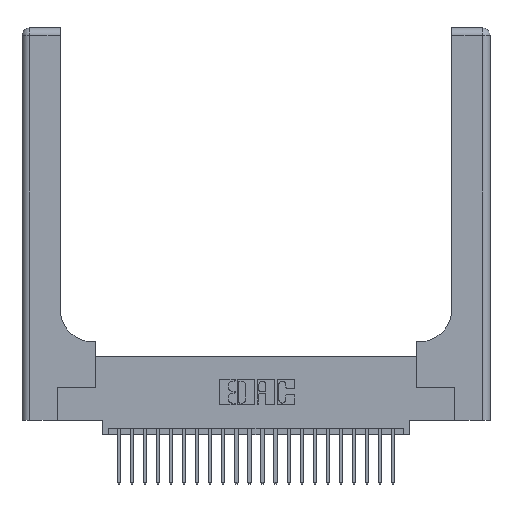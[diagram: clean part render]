
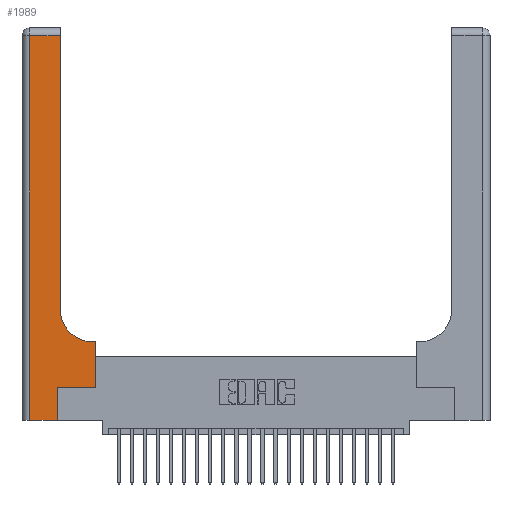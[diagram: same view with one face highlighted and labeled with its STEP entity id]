
A CAD part, top view. The second image highlights one B-rep face of the part: STEP entity #1989.
In plain terms, the highlighted planar face has unit normal (0, 0, 1).
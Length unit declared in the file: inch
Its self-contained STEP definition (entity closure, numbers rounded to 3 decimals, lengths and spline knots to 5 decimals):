
#318 = ORIENTED_EDGE ( 'NONE', *, *, #20393, .T. ) ;
#329 = CARTESIAN_POINT ( 'NONE',  ( 0.06, 0., 0.37 ) ) ;
#740 = EDGE_LOOP ( 'NONE', ( #21335, #24756, #16687, #18227, #22793, #7825, #9470, #23939, #318 ) ) ;
#787 = VECTOR ( 'NONE', #19542, 39.37008 ) ;
#1242 = VECTOR ( 'NONE', #10625, 39.37008 ) ;
#1989 = ADVANCED_FACE ( 'NONE', ( #13441 ), #8271, .F. ) ;
#2045 = LINE ( 'NONE', #21163, #17062 ) ;
#2426 = LINE ( 'NONE', #8465, #8575 ) ;
#2751 = VERTEX_POINT ( 'NONE', #9185 ) ;
#2783 = LINE ( 'NONE', #15528, #7411 ) ;
#2804 = EDGE_CURVE ( 'NONE', #16845, #6599, #2045, .T. ) ;
#3666 = CARTESIAN_POINT ( 'NONE',  ( 0.5585, 0.6, 0.37 ) ) ;
#4493 = EDGE_CURVE ( 'NONE', #8840, #17363, #17584, .T. ) ;
#4941 = EDGE_CURVE ( 'NONE', #7949, #16845, #2426, .T. ) ;
#5224 = VECTOR ( 'NONE', #7273, 39.37008 ) ;
#6599 = VERTEX_POINT ( 'NONE', #3666 ) ;
#6716 = DIRECTION ( 'NONE',  ( 0., 1., 0. ) ) ;
#7273 = DIRECTION ( 'NONE',  ( 0., -1., 0. ) ) ;
#7375 = EDGE_CURVE ( 'NONE', #10567, #2751, #8909, .T. ) ;
#7411 = VECTOR ( 'NONE', #21808, 39.37008 ) ;
#7825 = ORIENTED_EDGE ( 'NONE', *, *, #4941, .T. ) ;
#7949 = VERTEX_POINT ( 'NONE', #18211 ) ;
#8143 = LINE ( 'NONE', #21383, #787 ) ;
#8271 = PLANE ( 'NONE',  #23781 ) ;
#8465 = CARTESIAN_POINT ( 'NONE',  ( 0.269, 0.25, 0.37 ) ) ;
#8575 = VECTOR ( 'NONE', #18218, 39.37008 ) ;
#8693 = DIRECTION ( 'NONE',  ( 0., 0., -1. ) ) ;
#8840 = VERTEX_POINT ( 'NONE', #329 ) ;
#8909 = LINE ( 'NONE', #24203, #1242 ) ;
#9185 = CARTESIAN_POINT ( 'NONE',  ( 0.06, 2.94, 0.37 ) ) ;
#9470 = ORIENTED_EDGE ( 'NONE', *, *, #2804, .T. ) ;
#10244 = CARTESIAN_POINT ( 'NONE',  ( 0., 3., 0.37 ) ) ;
#10567 = VERTEX_POINT ( 'NONE', #21222 ) ;
#10625 = DIRECTION ( 'NONE',  ( -1., 0., 0. ) ) ;
#10696 = CARTESIAN_POINT ( 'NONE',  ( 0.269, 0., 0.37 ) ) ;
#12660 = CARTESIAN_POINT ( 'NONE',  ( 0., 0., 0.37 ) ) ;
#12858 = CARTESIAN_POINT ( 'NONE',  ( 0.5585, 0.25, 0.37 ) ) ;
#12900 = EDGE_CURVE ( 'NONE', #17363, #7949, #2783, .T. ) ;
#13174 = CARTESIAN_POINT ( 'NONE',  ( 0.06, 3., 0.37 ) ) ;
#13441 = FACE_OUTER_BOUND ( 'NONE', #740, .T. ) ;
#14233 = DIRECTION ( 'NONE',  ( 0., 0., -1. ) ) ;
#15145 = VECTOR ( 'NONE', #20596, 39.37008 ) ;
#15268 = LINE ( 'NONE', #18448, #17092 ) ;
#15528 = CARTESIAN_POINT ( 'NONE',  ( 0.269, 0., 0.37 ) ) ;
#16527 = EDGE_CURVE ( 'NONE', #6599, #24221, #8143, .T. ) ;
#16687 = ORIENTED_EDGE ( 'NONE', *, *, #18716, .T. ) ;
#16845 = VERTEX_POINT ( 'NONE', #12858 ) ;
#17062 = VECTOR ( 'NONE', #17097, 39.37008 ) ;
#17092 = VECTOR ( 'NONE', #6716, 39.37008 ) ;
#17097 = DIRECTION ( 'NONE',  ( 0., 1., 0. ) ) ;
#17363 = VERTEX_POINT ( 'NONE', #10696 ) ;
#17584 = LINE ( 'NONE', #12660, #15145 ) ;
#18211 = CARTESIAN_POINT ( 'NONE',  ( 0.269, 0.25, 0.37 ) ) ;
#18218 = DIRECTION ( 'NONE',  ( 1., 0., 0. ) ) ;
#18227 = ORIENTED_EDGE ( 'NONE', *, *, #4493, .T. ) ;
#18448 = CARTESIAN_POINT ( 'NONE',  ( 0.2915, 3., 0.37 ) ) ;
#18716 = EDGE_CURVE ( 'NONE', #2751, #8840, #25095, .T. ) ;
#18780 = AXIS2_PLACEMENT_3D ( 'NONE', #23960, #14233, #21905 ) ;
#19542 = DIRECTION ( 'NONE',  ( -1., 0., 0. ) ) ;
#20393 = EDGE_CURVE ( 'NONE', #24221, #23687, #23119, .T. ) ;
#20596 = DIRECTION ( 'NONE',  ( 1., 0., 0. ) ) ;
#21038 = CARTESIAN_POINT ( 'NONE',  ( 0.2915, 0.85, 0.37 ) ) ;
#21163 = CARTESIAN_POINT ( 'NONE',  ( 0.5585, 0.25, 0.37 ) ) ;
#21222 = CARTESIAN_POINT ( 'NONE',  ( 0.2915, 2.94, 0.37 ) ) ;
#21335 = ORIENTED_EDGE ( 'NONE', *, *, #24768, .T. ) ;
#21383 = CARTESIAN_POINT ( 'NONE',  ( 0.2915, 0.6, 0.37 ) ) ;
#21808 = DIRECTION ( 'NONE',  ( 0., 1., 0. ) ) ;
#21905 = DIRECTION ( 'NONE',  ( 1., 0., 0. ) ) ;
#22458 = CARTESIAN_POINT ( 'NONE',  ( 0.5415, 0.6, 0.37 ) ) ;
#22793 = ORIENTED_EDGE ( 'NONE', *, *, #12900, .T. ) ;
#23119 = CIRCLE ( 'NONE', #18780, 0.25 ) ;
#23687 = VERTEX_POINT ( 'NONE', #21038 ) ;
#23781 = AXIS2_PLACEMENT_3D ( 'NONE', #10244, #8693, #23878 ) ;
#23878 = DIRECTION ( 'NONE',  ( -1., 0., 0. ) ) ;
#23939 = ORIENTED_EDGE ( 'NONE', *, *, #16527, .T. ) ;
#23960 = CARTESIAN_POINT ( 'NONE',  ( 0.5415, 0.85, 0.37 ) ) ;
#24203 = CARTESIAN_POINT ( 'NONE',  ( 0., 2.94, 0.37 ) ) ;
#24221 = VERTEX_POINT ( 'NONE', #22458 ) ;
#24756 = ORIENTED_EDGE ( 'NONE', *, *, #7375, .T. ) ;
#24768 = EDGE_CURVE ( 'NONE', #23687, #10567, #15268, .T. ) ;
#25095 = LINE ( 'NONE', #13174, #5224 ) ;
